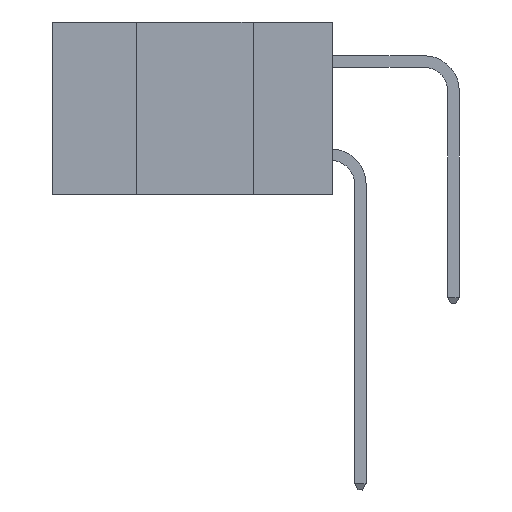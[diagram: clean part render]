
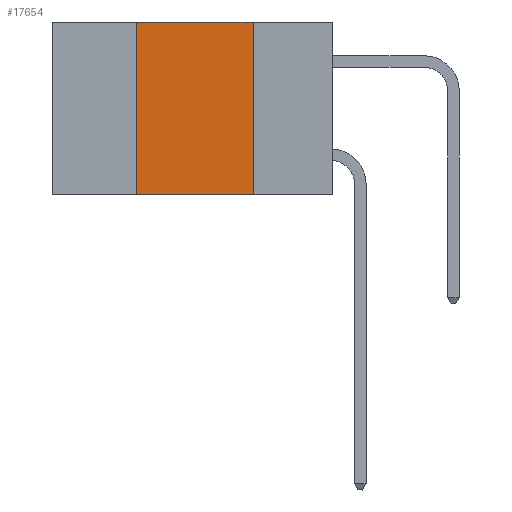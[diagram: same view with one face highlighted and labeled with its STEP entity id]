
A CAD part, left-side view. The second image highlights one B-rep face of the part: STEP entity #17654.
In plain terms, the highlighted planar face has unit normal (-1, 0, 0).
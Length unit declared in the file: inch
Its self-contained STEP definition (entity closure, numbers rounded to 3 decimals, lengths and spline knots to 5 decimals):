
#258 = EDGE_CURVE ( 'NONE', #4632, #5225, #16645, .T. ) ;
#765 = VECTOR ( 'NONE', #3319, 39.37008 ) ;
#840 = CARTESIAN_POINT ( 'NONE',  ( 0., 0.42, -0.37 ) ) ;
#2640 = DIRECTION ( 'NONE',  ( 0., 0., -1. ) ) ;
#2740 = LINE ( 'NONE', #8670, #6671 ) ;
#3050 = ORIENTED_EDGE ( 'NONE', *, *, #10357, .T. ) ;
#3319 = DIRECTION ( 'NONE',  ( 0., 0., 1. ) ) ;
#3688 = CARTESIAN_POINT ( 'NONE',  ( 0., 0.6, 0. ) ) ;
#3879 = DIRECTION ( 'NONE',  ( 0., 0., -1. ) ) ;
#4574 = CARTESIAN_POINT ( 'NONE',  ( 0., 0.17, 0. ) ) ;
#4632 = VERTEX_POINT ( 'NONE', #840 ) ;
#5225 = VERTEX_POINT ( 'NONE', #13029 ) ;
#5436 = DIRECTION ( 'NONE',  ( 1., 0., 0. ) ) ;
#6342 = LINE ( 'NONE', #10632, #6980 ) ;
#6671 = VECTOR ( 'NONE', #14589, 39.37008 ) ;
#6980 = VECTOR ( 'NONE', #10736, 39.37008 ) ;
#7057 = EDGE_CURVE ( 'NONE', #12172, #18316, #7187, .T. ) ;
#7187 = LINE ( 'NONE', #14581, #16210 ) ;
#7398 = ORIENTED_EDGE ( 'NONE', *, *, #17456, .F. ) ;
#8670 = CARTESIAN_POINT ( 'NONE',  ( 0., 0.6, 0. ) ) ;
#10357 = EDGE_CURVE ( 'NONE', #4632, #18316, #6342, .T. ) ;
#10632 = CARTESIAN_POINT ( 'NONE',  ( 0., 0.6, -0.37 ) ) ;
#10736 = DIRECTION ( 'NONE',  ( 0., -1., 0. ) ) ;
#11040 = AXIS2_PLACEMENT_3D ( 'NONE', #3688, #5436, #3879 ) ;
#11169 = FACE_OUTER_BOUND ( 'NONE', #12943, .T. ) ;
#12172 = VERTEX_POINT ( 'NONE', #4574 ) ;
#12943 = EDGE_LOOP ( 'NONE', ( #14782, #7398, #16349, #3050 ) ) ;
#13029 = CARTESIAN_POINT ( 'NONE',  ( 0., 0.42, 0. ) ) ;
#13103 = CARTESIAN_POINT ( 'NONE',  ( 0., 0.17, -0.37 ) ) ;
#14581 = CARTESIAN_POINT ( 'NONE',  ( 0., 0.17, -0.37 ) ) ;
#14589 = DIRECTION ( 'NONE',  ( 0., -1., 0. ) ) ;
#14782 = ORIENTED_EDGE ( 'NONE', *, *, #7057, .F. ) ;
#15752 = PLANE ( 'NONE',  #11040 ) ;
#16210 = VECTOR ( 'NONE', #2640, 39.37008 ) ;
#16349 = ORIENTED_EDGE ( 'NONE', *, *, #258, .F. ) ;
#16645 = LINE ( 'NONE', #16740, #765 ) ;
#16740 = CARTESIAN_POINT ( 'NONE',  ( 0., 0.42, -0.37 ) ) ;
#17456 = EDGE_CURVE ( 'NONE', #5225, #12172, #2740, .T. ) ;
#17654 = ADVANCED_FACE ( 'NONE', ( #11169 ), #15752, .F. ) ;
#18316 = VERTEX_POINT ( 'NONE', #13103 ) ;
